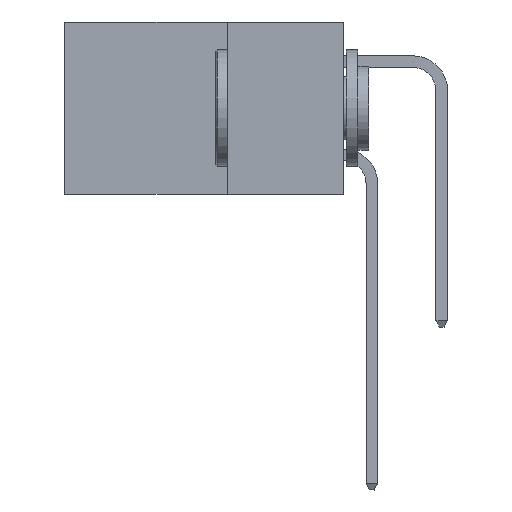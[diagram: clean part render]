
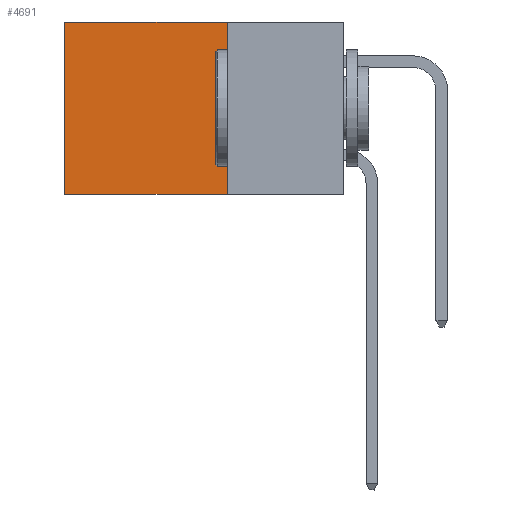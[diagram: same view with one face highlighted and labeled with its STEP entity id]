
A CAD part, left-side view. The second image highlights one B-rep face of the part: STEP entity #4691.
In plain terms, the highlighted planar face has unit normal (-1, 0, 0).
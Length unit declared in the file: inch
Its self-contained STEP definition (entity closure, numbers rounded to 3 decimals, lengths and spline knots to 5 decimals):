
#503 = DIRECTION ( 'NONE',  ( 1., 0., 0. ) ) ;
#913 = EDGE_CURVE ( 'NONE', #4401, #8425, #13406, .T. ) ;
#986 = CARTESIAN_POINT ( 'NONE',  ( 0.298, 0.25, -0.37 ) ) ;
#1474 = LINE ( 'NONE', #986, #4227 ) ;
#1627 = DIRECTION ( 'NONE',  ( 0., 0., -1. ) ) ;
#2400 = CARTESIAN_POINT ( 'NONE',  ( 0.298, 0.25, 0. ) ) ;
#2491 = CARTESIAN_POINT ( 'NONE',  ( 0.298, 0.25, 0. ) ) ;
#3102 = EDGE_CURVE ( 'NONE', #4350, #4401, #3598, .T. ) ;
#3220 = ORIENTED_EDGE ( 'NONE', *, *, #913, .T. ) ;
#3543 = ORIENTED_EDGE ( 'NONE', *, *, #6126, .F. ) ;
#3598 = LINE ( 'NONE', #2400, #11590 ) ;
#3795 = CARTESIAN_POINT ( 'NONE',  ( 0.298, 0.25, 0. ) ) ;
#4227 = VECTOR ( 'NONE', #8733, 39.37008 ) ;
#4350 = VERTEX_POINT ( 'NONE', #13365 ) ;
#4401 = VERTEX_POINT ( 'NONE', #9970 ) ;
#4691 = ADVANCED_FACE ( 'NONE', ( #4800 ), #6015, .F. ) ;
#4800 = FACE_OUTER_BOUND ( 'NONE', #11334, .T. ) ;
#5783 = DIRECTION ( 'NONE',  ( 0., 1., 0. ) ) ;
#6015 = PLANE ( 'NONE',  #9925 ) ;
#6102 = ORIENTED_EDGE ( 'NONE', *, *, #3102, .T. ) ;
#6126 = EDGE_CURVE ( 'NONE', #6861, #8425, #1474, .T. ) ;
#6861 = VERTEX_POINT ( 'NONE', #7228 ) ;
#7158 = ORIENTED_EDGE ( 'NONE', *, *, #8002, .F. ) ;
#7228 = CARTESIAN_POINT ( 'NONE',  ( 0.298, 0.25, -0.37 ) ) ;
#8002 = EDGE_CURVE ( 'NONE', #4350, #6861, #9385, .T. ) ;
#8425 = VERTEX_POINT ( 'NONE', #13358 ) ;
#8540 = VECTOR ( 'NONE', #13991, 39.37008 ) ;
#8733 = DIRECTION ( 'NONE',  ( 0., 1., 0. ) ) ;
#9385 = LINE ( 'NONE', #2491, #12697 ) ;
#9925 = AXIS2_PLACEMENT_3D ( 'NONE', #3795, #503, #1627 ) ;
#9970 = CARTESIAN_POINT ( 'NONE',  ( 0.298, 0.6, 0. ) ) ;
#11334 = EDGE_LOOP ( 'NONE', ( #3220, #3543, #7158, #6102 ) ) ;
#11590 = VECTOR ( 'NONE', #5783, 39.37008 ) ;
#12529 = DIRECTION ( 'NONE',  ( 0., 0., -1. ) ) ;
#12697 = VECTOR ( 'NONE', #12529, 39.37008 ) ;
#13358 = CARTESIAN_POINT ( 'NONE',  ( 0.298, 0.6, -0.37 ) ) ;
#13365 = CARTESIAN_POINT ( 'NONE',  ( 0.298, 0.25, 0. ) ) ;
#13406 = LINE ( 'NONE', #13846, #8540 ) ;
#13846 = CARTESIAN_POINT ( 'NONE',  ( 0.298, 0.6, 0. ) ) ;
#13991 = DIRECTION ( 'NONE',  ( 0., 0., -1. ) ) ;
